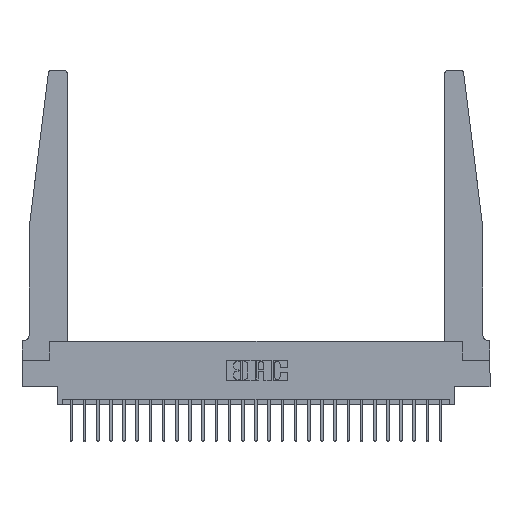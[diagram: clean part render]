
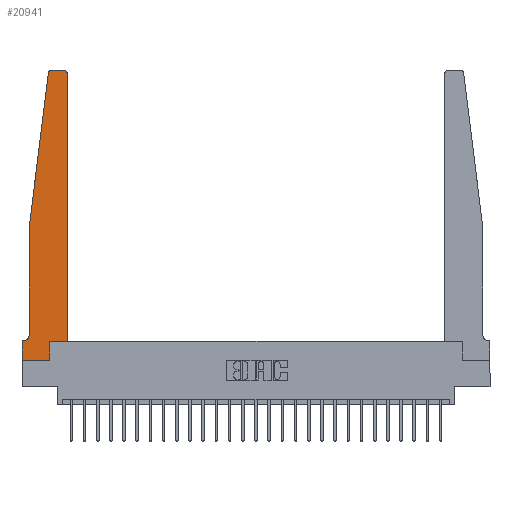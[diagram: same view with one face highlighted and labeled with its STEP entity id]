
A CAD part, top view. The second image highlights one B-rep face of the part: STEP entity #20941.
In plain terms, the highlighted planar face has unit normal (0, 0, 1).
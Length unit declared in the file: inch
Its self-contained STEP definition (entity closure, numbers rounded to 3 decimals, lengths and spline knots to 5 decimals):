
#127 = VECTOR ( 'NONE', #186, 39.37008 ) ;
#186 = DIRECTION ( 'NONE',  ( 0., -1., 0. ) ) ;
#190 = DIRECTION ( 'NONE',  ( 1., 0., 0. ) ) ;
#577 = DIRECTION ( 'NONE',  ( 0., 0., 1. ) ) ;
#1128 = LINE ( 'NONE', #1386, #3851 ) ;
#1310 = DIRECTION ( 'NONE',  ( 0., 0., 1. ) ) ;
#1385 = ORIENTED_EDGE ( 'NONE', *, *, #3214, .T. ) ;
#1386 = CARTESIAN_POINT ( 'NONE',  ( 0.065, 1.25, 0.37 ) ) ;
#1524 = VERTEX_POINT ( 'NONE', #23306 ) ;
#1882 = VERTEX_POINT ( 'NONE', #10414 ) ;
#1934 = CARTESIAN_POINT ( 'NONE',  ( 0.065, 0.1875, 0.37 ) ) ;
#2230 = VERTEX_POINT ( 'NONE', #22129 ) ;
#2896 = CARTESIAN_POINT ( 'NONE',  ( 0.2605, 0.18, 0.37 ) ) ;
#3141 = VERTEX_POINT ( 'NONE', #9115 ) ;
#3214 = EDGE_CURVE ( 'NONE', #5966, #16686, #22634, .T. ) ;
#3601 = CARTESIAN_POINT ( 'NONE',  ( 0., 0., 0.37 ) ) ;
#3851 = VECTOR ( 'NONE', #23429, 39.37008 ) ;
#3861 = LINE ( 'NONE', #3601, #127 ) ;
#4191 = EDGE_LOOP ( 'NONE', ( #1385, #19087, #24798, #18666, #18922, #4424, #20202, #16157, #18575, #5035, #22968, #4313 ) ) ;
#4313 = ORIENTED_EDGE ( 'NONE', *, *, #19334, .T. ) ;
#4424 = ORIENTED_EDGE ( 'NONE', *, *, #24267, .T. ) ;
#4724 = DIRECTION ( 'NONE',  ( 0., 1., 0. ) ) ;
#4753 = PLANE ( 'NONE',  #10098 ) ;
#4819 = VERTEX_POINT ( 'NONE', #2896 ) ;
#5035 = ORIENTED_EDGE ( 'NONE', *, *, #23608, .T. ) ;
#5508 = CARTESIAN_POINT ( 'NONE',  ( 0.395, 2.75, 0.37 ) ) ;
#5910 = EDGE_CURVE ( 'NONE', #2230, #4819, #22691, .T. ) ;
#5966 = VERTEX_POINT ( 'NONE', #5508 ) ;
#6253 = CARTESIAN_POINT ( 'NONE',  ( 0.395, 2.72, 0.37 ) ) ;
#6268 = EDGE_CURVE ( 'NONE', #3141, #2230, #20238, .T. ) ;
#6391 = DIRECTION ( 'NONE',  ( -1., 0., 0. ) ) ;
#6481 = DIRECTION ( 'NONE',  ( 0., -1., 0. ) ) ;
#6984 = CARTESIAN_POINT ( 'NONE',  ( 0.2605, 0.18, 0.37 ) ) ;
#7419 = VERTEX_POINT ( 'NONE', #8952 ) ;
#7700 = CIRCLE ( 'NONE', #24093, 0.03 ) ;
#7816 = VECTOR ( 'NONE', #4724, 39.37008 ) ;
#8343 = DIRECTION ( 'NONE',  ( 0., 0., 1. ) ) ;
#8952 = CARTESIAN_POINT ( 'NONE',  ( 0.015, 0.1875, 0.37 ) ) ;
#8999 = DIRECTION ( 'NONE',  ( 1., 0., 0. ) ) ;
#9115 = CARTESIAN_POINT ( 'NONE',  ( 0., 0., 0.37 ) ) ;
#10036 = DIRECTION ( 'NONE',  ( -1., 0., 0. ) ) ;
#10098 = AXIS2_PLACEMENT_3D ( 'NONE', #12857, #8343, #16544 ) ;
#10232 = VECTOR ( 'NONE', #6481, 39.37008 ) ;
#10308 = CIRCLE ( 'NONE', #17049, 0.03 ) ;
#10414 = CARTESIAN_POINT ( 'NONE',  ( 0.425, 0.18, 0.37 ) ) ;
#10474 = CARTESIAN_POINT ( 'NONE',  ( 0.065, 1.25, 0.37 ) ) ;
#11016 = CARTESIAN_POINT ( 'NONE',  ( 0.425, 0.18, 0.37 ) ) ;
#11306 = CARTESIAN_POINT ( 'NONE',  ( 0.24675, 2.72367, 0.37 ) ) ;
#11632 = CARTESIAN_POINT ( 'NONE',  ( 0.425, 0.18, 0.37 ) ) ;
#12756 = CARTESIAN_POINT ( 'NONE',  ( 0.425, 2.72, 0.37 ) ) ;
#12857 = CARTESIAN_POINT ( 'NONE',  ( 0., 0.1875, 0.37 ) ) ;
#12922 = EDGE_CURVE ( 'NONE', #19397, #1524, #24398, .T. ) ;
#13646 = EDGE_CURVE ( 'NONE', #16686, #19580, #7700, .T. ) ;
#14439 = CARTESIAN_POINT ( 'NONE',  ( 0.015, 0.2375, 0.37 ) ) ;
#14886 = EDGE_CURVE ( 'NONE', #18244, #3141, #3861, .T. ) ;
#15554 = EDGE_CURVE ( 'NONE', #1524, #7419, #19421, .T. ) ;
#15983 = EDGE_CURVE ( 'NONE', #19580, #19397, #1128, .T. ) ;
#16157 = ORIENTED_EDGE ( 'NONE', *, *, #6268, .T. ) ;
#16544 = DIRECTION ( 'NONE',  ( 1., 0., 0. ) ) ;
#16555 = DIRECTION ( 'NONE',  ( 1., 0., 0. ) ) ;
#16686 = VERTEX_POINT ( 'NONE', #21826 ) ;
#17049 = AXIS2_PLACEMENT_3D ( 'NONE', #6253, #577, #20761 ) ;
#18150 = AXIS2_PLACEMENT_3D ( 'NONE', #14439, #20467, #22485 ) ;
#18244 = VERTEX_POINT ( 'NONE', #22367 ) ;
#18295 = CARTESIAN_POINT ( 'NONE',  ( 0., 0., 0.37 ) ) ;
#18575 = ORIENTED_EDGE ( 'NONE', *, *, #5910, .T. ) ;
#18666 = ORIENTED_EDGE ( 'NONE', *, *, #12922, .T. ) ;
#18922 = ORIENTED_EDGE ( 'NONE', *, *, #15554, .T. ) ;
#19087 = ORIENTED_EDGE ( 'NONE', *, *, #13646, .T. ) ;
#19334 = EDGE_CURVE ( 'NONE', #19452, #5966, #10308, .T. ) ;
#19397 = VERTEX_POINT ( 'NONE', #20489 ) ;
#19421 = CIRCLE ( 'NONE', #18150, 0.05 ) ;
#19452 = VERTEX_POINT ( 'NONE', #12756 ) ;
#19580 = VERTEX_POINT ( 'NONE', #11306 ) ;
#19855 = DIRECTION ( 'NONE',  ( 0., 1., 0. ) ) ;
#20202 = ORIENTED_EDGE ( 'NONE', *, *, #14886, .T. ) ;
#20238 = LINE ( 'NONE', #18295, #25072 ) ;
#20467 = DIRECTION ( 'NONE',  ( 0., 0., -1. ) ) ;
#20489 = CARTESIAN_POINT ( 'NONE',  ( 0.065, 1.25, 0.37 ) ) ;
#20761 = DIRECTION ( 'NONE',  ( 1., 0., 0. ) ) ;
#20941 = ADVANCED_FACE ( 'NONE', ( #22596 ), #4753, .T. ) ;
#21171 = VECTOR ( 'NONE', #6391, 39.37008 ) ;
#21240 = CARTESIAN_POINT ( 'NONE',  ( 0.27653, 2.72, 0.37 ) ) ;
#21285 = VECTOR ( 'NONE', #16555, 39.37008 ) ;
#21826 = CARTESIAN_POINT ( 'NONE',  ( 0.27653, 2.75, 0.37 ) ) ;
#22129 = CARTESIAN_POINT ( 'NONE',  ( 0.2605, 0., 0.37 ) ) ;
#22132 = LINE ( 'NONE', #11632, #22136 ) ;
#22136 = VECTOR ( 'NONE', #19855, 39.37008 ) ;
#22367 = CARTESIAN_POINT ( 'NONE',  ( 0., 0.1875, 0.37 ) ) ;
#22485 = DIRECTION ( 'NONE',  ( -1., 0., 0. ) ) ;
#22596 = FACE_OUTER_BOUND ( 'NONE', #4191, .T. ) ;
#22604 = LINE ( 'NONE', #11016, #21285 ) ;
#22634 = LINE ( 'NONE', #24436, #21171 ) ;
#22691 = LINE ( 'NONE', #6984, #7816 ) ;
#22968 = ORIENTED_EDGE ( 'NONE', *, *, #24805, .T. ) ;
#23306 = CARTESIAN_POINT ( 'NONE',  ( 0.065, 0.2375, 0.37 ) ) ;
#23354 = VECTOR ( 'NONE', #10036, 39.37008 ) ;
#23429 = DIRECTION ( 'NONE',  ( -0.122, -0.992, 0. ) ) ;
#23608 = EDGE_CURVE ( 'NONE', #4819, #1882, #22604, .T. ) ;
#23720 = LINE ( 'NONE', #1934, #23354 ) ;
#24093 = AXIS2_PLACEMENT_3D ( 'NONE', #21240, #1310, #8999 ) ;
#24267 = EDGE_CURVE ( 'NONE', #7419, #18244, #23720, .T. ) ;
#24398 = LINE ( 'NONE', #10474, #10232 ) ;
#24436 = CARTESIAN_POINT ( 'NONE',  ( 0.25, 2.75, 0.37 ) ) ;
#24798 = ORIENTED_EDGE ( 'NONE', *, *, #15983, .T. ) ;
#24805 = EDGE_CURVE ( 'NONE', #1882, #19452, #22132, .T. ) ;
#25072 = VECTOR ( 'NONE', #190, 39.37008 ) ;
